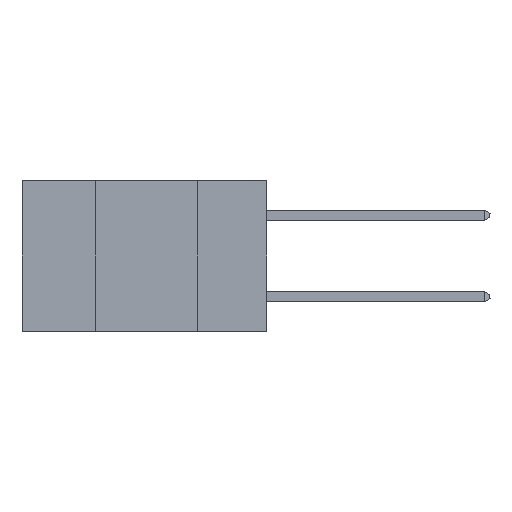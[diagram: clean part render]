
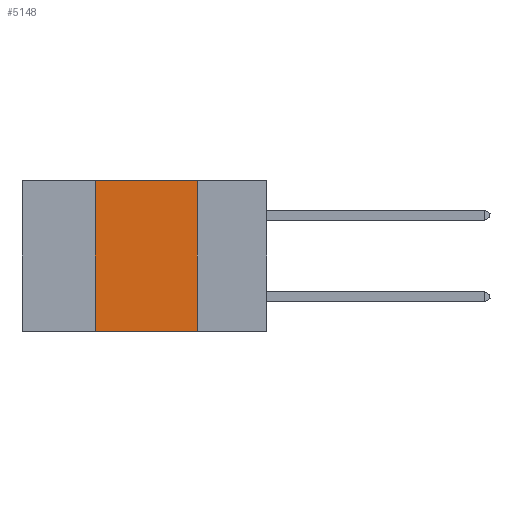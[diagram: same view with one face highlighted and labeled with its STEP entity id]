
A CAD part, left-side view. The second image highlights one B-rep face of the part: STEP entity #5148.
In plain terms, the highlighted planar face has unit normal (-1, 0, 0).
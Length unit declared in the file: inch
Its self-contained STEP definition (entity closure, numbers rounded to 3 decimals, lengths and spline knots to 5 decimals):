
#92 = VECTOR ( 'NONE', #7050, 39.37008 ) ;
#508 = CARTESIAN_POINT ( 'NONE',  ( 0., 0.17, -0.37 ) ) ;
#670 = PLANE ( 'NONE',  #5403 ) ;
#948 = CARTESIAN_POINT ( 'NONE',  ( 0., 0.6, 0. ) ) ;
#968 = DIRECTION ( 'NONE',  ( 1., 0., 0. ) ) ;
#1012 = DIRECTION ( 'NONE',  ( 0., 0., -1. ) ) ;
#1047 = CARTESIAN_POINT ( 'NONE',  ( 0., 0.6, -0.37 ) ) ;
#1398 = VERTEX_POINT ( 'NONE', #10574 ) ;
#1468 = CARTESIAN_POINT ( 'NONE',  ( 0., 0.17, 0. ) ) ;
#2042 = EDGE_CURVE ( 'NONE', #18144, #16984, #8589, .T. ) ;
#4108 = EDGE_LOOP ( 'NONE', ( #9750, #8895, #16674, #12159 ) ) ;
#5148 = ADVANCED_FACE ( 'NONE', ( #7920 ), #670, .F. ) ;
#5403 = AXIS2_PLACEMENT_3D ( 'NONE', #948, #968, #1012 ) ;
#7050 = DIRECTION ( 'NONE',  ( 0., 0., -1. ) ) ;
#7273 = EDGE_CURVE ( 'NONE', #11560, #18144, #16720, .T. ) ;
#7477 = EDGE_CURVE ( 'NONE', #1398, #16984, #9975, .T. ) ;
#7687 = DIRECTION ( 'NONE',  ( 0., -1., 0. ) ) ;
#7920 = FACE_OUTER_BOUND ( 'NONE', #4108, .T. ) ;
#8053 = DIRECTION ( 'NONE',  ( 0., -1., 0. ) ) ;
#8589 = LINE ( 'NONE', #1468, #92 ) ;
#8895 = ORIENTED_EDGE ( 'NONE', *, *, #7273, .F. ) ;
#9357 = VECTOR ( 'NONE', #7687, 39.37008 ) ;
#9750 = ORIENTED_EDGE ( 'NONE', *, *, #2042, .F. ) ;
#9975 = LINE ( 'NONE', #1047, #13287 ) ;
#10574 = CARTESIAN_POINT ( 'NONE',  ( 0., 0.42, -0.37 ) ) ;
#11560 = VERTEX_POINT ( 'NONE', #17927 ) ;
#11707 = EDGE_CURVE ( 'NONE', #1398, #11560, #15686, .T. ) ;
#11738 = CARTESIAN_POINT ( 'NONE',  ( 0., 0.17, 0. ) ) ;
#12009 = VECTOR ( 'NONE', #14150, 39.37008 ) ;
#12159 = ORIENTED_EDGE ( 'NONE', *, *, #7477, .T. ) ;
#12769 = CARTESIAN_POINT ( 'NONE',  ( 0., 0.42, 0. ) ) ;
#13287 = VECTOR ( 'NONE', #8053, 39.37008 ) ;
#14150 = DIRECTION ( 'NONE',  ( 0., 0., 1. ) ) ;
#15686 = LINE ( 'NONE', #12769, #12009 ) ;
#16674 = ORIENTED_EDGE ( 'NONE', *, *, #11707, .F. ) ;
#16720 = LINE ( 'NONE', #17314, #9357 ) ;
#16984 = VERTEX_POINT ( 'NONE', #508 ) ;
#17314 = CARTESIAN_POINT ( 'NONE',  ( 0., 0.6, 0. ) ) ;
#17927 = CARTESIAN_POINT ( 'NONE',  ( 0., 0.42, 0. ) ) ;
#18144 = VERTEX_POINT ( 'NONE', #11738 ) ;
